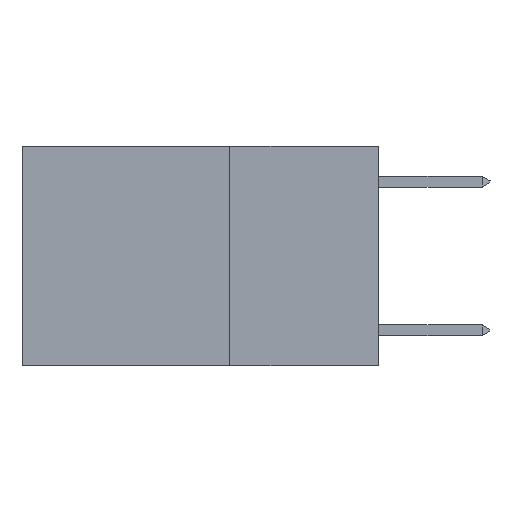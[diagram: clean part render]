
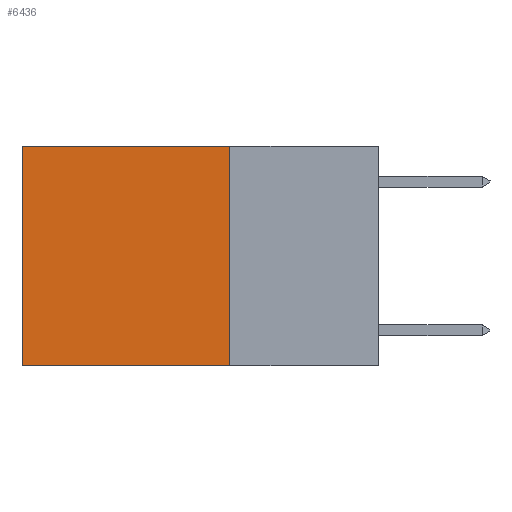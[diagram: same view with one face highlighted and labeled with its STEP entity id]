
A CAD part, left-side view. The second image highlights one B-rep face of the part: STEP entity #6436.
In plain terms, the highlighted planar face has unit normal (-1, 0, 0).
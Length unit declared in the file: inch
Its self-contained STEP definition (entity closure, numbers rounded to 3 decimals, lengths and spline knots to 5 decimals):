
#699 = DIRECTION ( 'NONE',  ( 0., 0., -1. ) ) ;
#1578 = EDGE_CURVE ( 'NONE', #6694, #5290, #4331, .T. ) ;
#1685 = ORIENTED_EDGE ( 'NONE', *, *, #1749, .T. ) ;
#1749 = EDGE_CURVE ( 'NONE', #3933, #8806, #3392, .T. ) ;
#2131 = EDGE_CURVE ( 'NONE', #6694, #3933, #3136, .T. ) ;
#2148 = CARTESIAN_POINT ( 'NONE',  ( 0.2625, 0.25, -0.37 ) ) ;
#2348 = VECTOR ( 'NONE', #3245, 39.37008 ) ;
#2504 = EDGE_LOOP ( 'NONE', ( #1685, #8973, #7224, #3441 ) ) ;
#3136 = LINE ( 'NONE', #3882, #3385 ) ;
#3245 = DIRECTION ( 'NONE',  ( 0., 0., -1. ) ) ;
#3309 = FACE_OUTER_BOUND ( 'NONE', #2504, .T. ) ;
#3385 = VECTOR ( 'NONE', #5156, 39.37008 ) ;
#3392 = LINE ( 'NONE', #7557, #5096 ) ;
#3441 = ORIENTED_EDGE ( 'NONE', *, *, #2131, .T. ) ;
#3555 = AXIS2_PLACEMENT_3D ( 'NONE', #9176, #5104, #699 ) ;
#3882 = CARTESIAN_POINT ( 'NONE',  ( 0.2625, 0.25, 0. ) ) ;
#3933 = VERTEX_POINT ( 'NONE', #4149 ) ;
#4045 = CARTESIAN_POINT ( 'NONE',  ( 0.2625, 0.25, 0. ) ) ;
#4149 = CARTESIAN_POINT ( 'NONE',  ( 0.2625, 0.6, 0. ) ) ;
#4331 = LINE ( 'NONE', #4045, #2348 ) ;
#4489 = CARTESIAN_POINT ( 'NONE',  ( 0.2625, 0.6, -0.37 ) ) ;
#4915 = CARTESIAN_POINT ( 'NONE',  ( 0.2625, 0.25, -0.37 ) ) ;
#4919 = DIRECTION ( 'NONE',  ( 0., 0., -1. ) ) ;
#5075 = EDGE_CURVE ( 'NONE', #5290, #8806, #6046, .T. ) ;
#5078 = PLANE ( 'NONE',  #3555 ) ;
#5096 = VECTOR ( 'NONE', #4919, 39.37008 ) ;
#5104 = DIRECTION ( 'NONE',  ( 1., 0., 0. ) ) ;
#5156 = DIRECTION ( 'NONE',  ( 0., 1., 0. ) ) ;
#5290 = VERTEX_POINT ( 'NONE', #2148 ) ;
#6046 = LINE ( 'NONE', #4915, #7637 ) ;
#6436 = ADVANCED_FACE ( 'NONE', ( #3309 ), #5078, .F. ) ;
#6694 = VERTEX_POINT ( 'NONE', #8075 ) ;
#7024 = DIRECTION ( 'NONE',  ( 0., 1., 0. ) ) ;
#7224 = ORIENTED_EDGE ( 'NONE', *, *, #1578, .F. ) ;
#7557 = CARTESIAN_POINT ( 'NONE',  ( 0.2625, 0.6, 0. ) ) ;
#7637 = VECTOR ( 'NONE', #7024, 39.37008 ) ;
#8075 = CARTESIAN_POINT ( 'NONE',  ( 0.2625, 0.25, 0. ) ) ;
#8806 = VERTEX_POINT ( 'NONE', #4489 ) ;
#8973 = ORIENTED_EDGE ( 'NONE', *, *, #5075, .F. ) ;
#9176 = CARTESIAN_POINT ( 'NONE',  ( 0.2625, 0.25, 0. ) ) ;
